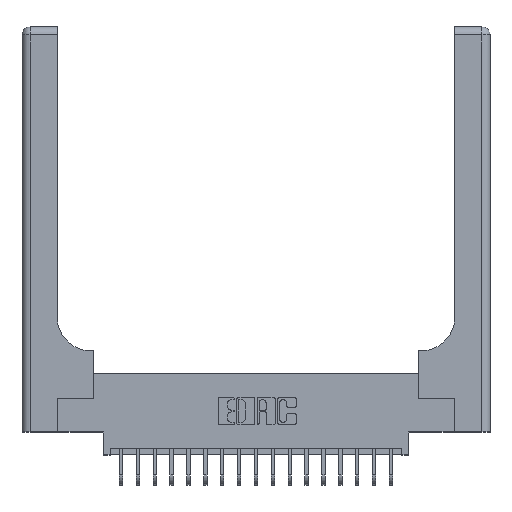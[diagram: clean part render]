
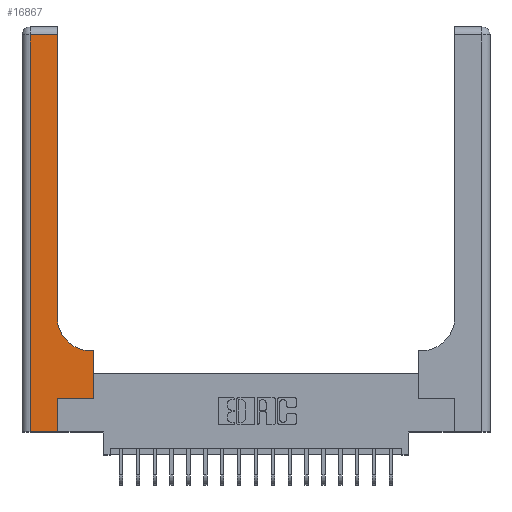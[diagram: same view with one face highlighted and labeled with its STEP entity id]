
A CAD part, top view. The second image highlights one B-rep face of the part: STEP entity #16867.
In plain terms, the highlighted planar face has unit normal (0, 0, 1).
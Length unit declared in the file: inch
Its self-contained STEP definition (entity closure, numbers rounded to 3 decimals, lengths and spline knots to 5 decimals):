
#192 = CARTESIAN_POINT ( 'NONE',  ( 0.06, 0., 0.37 ) ) ;
#261 = ORIENTED_EDGE ( 'NONE', *, *, #9548, .T. ) ;
#478 = LINE ( 'NONE', #6005, #13841 ) ;
#601 = PLANE ( 'NONE',  #18957 ) ;
#747 = VECTOR ( 'NONE', #10803, 39.37008 ) ;
#1286 = AXIS2_PLACEMENT_3D ( 'NONE', #14967, #2966, #21530 ) ;
#1689 = CARTESIAN_POINT ( 'NONE',  ( 0.06, 3., 0.37 ) ) ;
#2403 = CARTESIAN_POINT ( 'NONE',  ( 0.26, 2.94, 0.37 ) ) ;
#2448 = VECTOR ( 'NONE', #16917, 39.37008 ) ;
#2853 = VERTEX_POINT ( 'NONE', #3266 ) ;
#2896 = EDGE_LOOP ( 'NONE', ( #17977, #4524, #6426, #7406, #19126, #21149, #6049, #13557, #261 ) ) ;
#2949 = VECTOR ( 'NONE', #10141, 39.37008 ) ;
#2966 = DIRECTION ( 'NONE',  ( 0., 0., -1. ) ) ;
#3253 = CARTESIAN_POINT ( 'NONE',  ( 0.26, 0.85, 0.37 ) ) ;
#3266 = CARTESIAN_POINT ( 'NONE',  ( 0.265, 0., 0.37 ) ) ;
#3760 = LINE ( 'NONE', #16286, #14251 ) ;
#3938 = LINE ( 'NONE', #14777, #17792 ) ;
#4383 = EDGE_CURVE ( 'NONE', #8165, #15494, #12275, .T. ) ;
#4524 = ORIENTED_EDGE ( 'NONE', *, *, #4383, .T. ) ;
#6005 = CARTESIAN_POINT ( 'NONE',  ( 0., 0., 0.37 ) ) ;
#6049 = ORIENTED_EDGE ( 'NONE', *, *, #13911, .T. ) ;
#6386 = EDGE_CURVE ( 'NONE', #9537, #8165, #8743, .T. ) ;
#6426 = ORIENTED_EDGE ( 'NONE', *, *, #17581, .T. ) ;
#6519 = CARTESIAN_POINT ( 'NONE',  ( 0.528, 0.25, 0.37 ) ) ;
#7057 = FACE_OUTER_BOUND ( 'NONE', #2896, .T. ) ;
#7406 = ORIENTED_EDGE ( 'NONE', *, *, #16549, .T. ) ;
#7625 = DIRECTION ( 'NONE',  ( 1., 0., 0. ) ) ;
#8165 = VERTEX_POINT ( 'NONE', #2403 ) ;
#8457 = VERTEX_POINT ( 'NONE', #9869 ) ;
#8743 = LINE ( 'NONE', #18514, #2448 ) ;
#8897 = EDGE_CURVE ( 'NONE', #11970, #10566, #3938, .T. ) ;
#9257 = LINE ( 'NONE', #16207, #17585 ) ;
#9537 = VERTEX_POINT ( 'NONE', #3253 ) ;
#9548 = EDGE_CURVE ( 'NONE', #10566, #9537, #19813, .T. ) ;
#9809 = DIRECTION ( 'NONE',  ( 0., 1., 0. ) ) ;
#9869 = CARTESIAN_POINT ( 'NONE',  ( 0.265, 0.25, 0.37 ) ) ;
#10056 = CARTESIAN_POINT ( 'NONE',  ( 0.06, 2.94, 0.37 ) ) ;
#10141 = DIRECTION ( 'NONE',  ( 0., 1., 0. ) ) ;
#10566 = VERTEX_POINT ( 'NONE', #21561 ) ;
#10803 = DIRECTION ( 'NONE',  ( -1., 0., 0. ) ) ;
#11970 = VERTEX_POINT ( 'NONE', #18012 ) ;
#12275 = LINE ( 'NONE', #20730, #747 ) ;
#12310 = CARTESIAN_POINT ( 'NONE',  ( 0., 3., 0.37 ) ) ;
#12944 = DIRECTION ( 'NONE',  ( -1., 0., 0. ) ) ;
#13557 = ORIENTED_EDGE ( 'NONE', *, *, #8897, .T. ) ;
#13841 = VECTOR ( 'NONE', #7625, 39.37008 ) ;
#13911 = EDGE_CURVE ( 'NONE', #16728, #11970, #3760, .T. ) ;
#14251 = VECTOR ( 'NONE', #9809, 39.37008 ) ;
#14499 = EDGE_CURVE ( 'NONE', #2853, #8457, #19636, .T. ) ;
#14608 = DIRECTION ( 'NONE',  ( 1., 0., 0. ) ) ;
#14777 = CARTESIAN_POINT ( 'NONE',  ( 0.26, 0.6, 0.37 ) ) ;
#14782 = EDGE_CURVE ( 'NONE', #8457, #16728, #9257, .T. ) ;
#14967 = CARTESIAN_POINT ( 'NONE',  ( 0.51, 0.85, 0.37 ) ) ;
#15375 = DIRECTION ( 'NONE',  ( -1., 0., 0. ) ) ;
#15494 = VERTEX_POINT ( 'NONE', #10056 ) ;
#16207 = CARTESIAN_POINT ( 'NONE',  ( 0.265, 0.25, 0.37 ) ) ;
#16286 = CARTESIAN_POINT ( 'NONE',  ( 0.528, 0.25, 0.37 ) ) ;
#16525 = DIRECTION ( 'NONE',  ( 0., -1., 0. ) ) ;
#16549 = EDGE_CURVE ( 'NONE', #19713, #2853, #478, .T. ) ;
#16728 = VERTEX_POINT ( 'NONE', #6519 ) ;
#16750 = CARTESIAN_POINT ( 'NONE',  ( 0.265, 0., 0.37 ) ) ;
#16867 = ADVANCED_FACE ( 'NONE', ( #7057 ), #601, .F. ) ;
#16917 = DIRECTION ( 'NONE',  ( 0., 1., 0. ) ) ;
#17581 = EDGE_CURVE ( 'NONE', #15494, #19713, #19768, .T. ) ;
#17585 = VECTOR ( 'NONE', #14608, 39.37008 ) ;
#17792 = VECTOR ( 'NONE', #12944, 39.37008 ) ;
#17950 = VECTOR ( 'NONE', #16525, 39.37008 ) ;
#17977 = ORIENTED_EDGE ( 'NONE', *, *, #6386, .T. ) ;
#18012 = CARTESIAN_POINT ( 'NONE',  ( 0.528, 0.6, 0.37 ) ) ;
#18514 = CARTESIAN_POINT ( 'NONE',  ( 0.26, 3., 0.37 ) ) ;
#18957 = AXIS2_PLACEMENT_3D ( 'NONE', #12310, #20369, #15375 ) ;
#19126 = ORIENTED_EDGE ( 'NONE', *, *, #14499, .T. ) ;
#19636 = LINE ( 'NONE', #16750, #2949 ) ;
#19713 = VERTEX_POINT ( 'NONE', #192 ) ;
#19768 = LINE ( 'NONE', #1689, #17950 ) ;
#19813 = CIRCLE ( 'NONE', #1286, 0.25 ) ;
#20369 = DIRECTION ( 'NONE',  ( 0., 0., -1. ) ) ;
#20730 = CARTESIAN_POINT ( 'NONE',  ( 0., 2.94, 0.37 ) ) ;
#21149 = ORIENTED_EDGE ( 'NONE', *, *, #14782, .T. ) ;
#21530 = DIRECTION ( 'NONE',  ( 1., 0., 0. ) ) ;
#21561 = CARTESIAN_POINT ( 'NONE',  ( 0.51, 0.6, 0.37 ) ) ;
